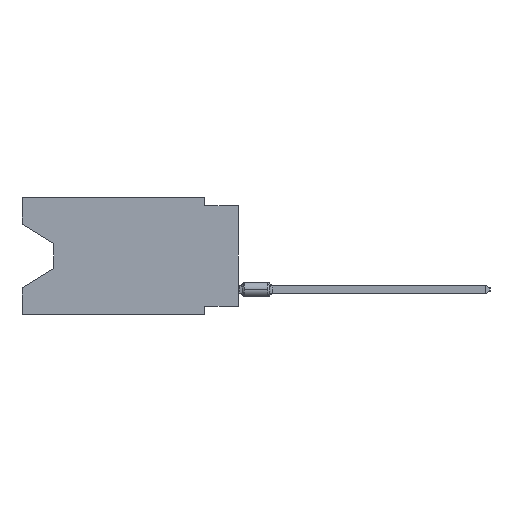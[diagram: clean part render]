
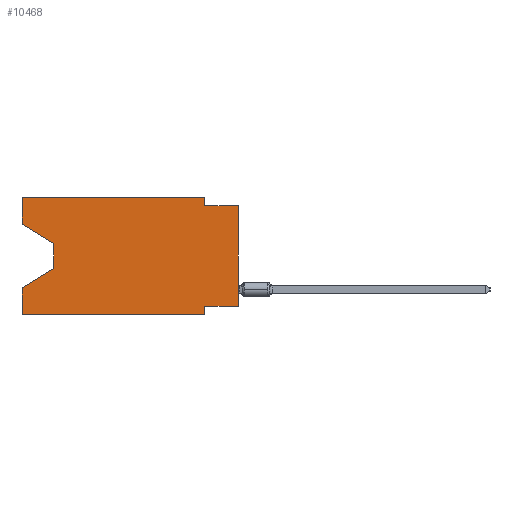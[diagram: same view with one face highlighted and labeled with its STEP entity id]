
A CAD part, left-side view. The second image highlights one B-rep face of the part: STEP entity #10468.
In plain terms, the highlighted planar face has unit normal (-1, 0, 0).
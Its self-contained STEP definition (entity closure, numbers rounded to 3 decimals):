
#1306 = EDGE_CURVE ( 'NONE', #19999, #4878, #35675, .T. ) ;
#1362 = DIRECTION ( 'NONE',  ( 0., 0., -1. ) ) ;
#1795 = VERTEX_POINT ( 'NONE', #6990 ) ;
#1924 = LINE ( 'NONE', #17501, #7468 ) ;
#2121 = DIRECTION ( 'NONE',  ( 0., 0., -1. ) ) ;
#3189 = CARTESIAN_POINT ( 'NONE',  ( 0., 0., 0. ) ) ;
#3445 = VERTEX_POINT ( 'NONE', #20941 ) ;
#3462 = LINE ( 'NONE', #12535, #15370 ) ;
#3590 = EDGE_CURVE ( 'NONE', #22829, #10053, #12602, .T. ) ;
#3717 = CARTESIAN_POINT ( 'NONE',  ( 0., 16.383, -8.89 ) ) ;
#4455 = LINE ( 'NONE', #10248, #30236 ) ;
#4628 = ORIENTED_EDGE ( 'NONE', *, *, #26332, .F. ) ;
#4878 = VERTEX_POINT ( 'NONE', #6322 ) ;
#4964 = EDGE_CURVE ( 'NONE', #11980, #38123, #12509, .T. ) ;
#5259 = CARTESIAN_POINT ( 'NONE',  ( 0., 2.54, -8.89 ) ) ;
#6066 = DIRECTION ( 'NONE',  ( 0., 0., 1. ) ) ;
#6203 = CARTESIAN_POINT ( 'NONE',  ( 0., 16.383, 0. ) ) ;
#6322 = CARTESIAN_POINT ( 'NONE',  ( 0., 0., -0.635 ) ) ;
#6726 = ORIENTED_EDGE ( 'NONE', *, *, #31662, .T. ) ;
#6990 = CARTESIAN_POINT ( 'NONE',  ( 0., 13.97, -5.385 ) ) ;
#6999 = DIRECTION ( 'NONE',  ( 0., -0.855, -0.519 ) ) ;
#7286 = CARTESIAN_POINT ( 'NONE',  ( 0., 16.383, -8.89 ) ) ;
#7453 = EDGE_CURVE ( 'NONE', #12518, #3445, #3462, .T. ) ;
#7468 = VECTOR ( 'NONE', #13704, 1000. ) ;
#7563 = CARTESIAN_POINT ( 'NONE',  ( 0., 16.383, 0. ) ) ;
#7879 = EDGE_CURVE ( 'NONE', #3445, #4878, #4455, .T. ) ;
#8936 = DIRECTION ( 'NONE',  ( 0., -1., 0. ) ) ;
#9057 = DIRECTION ( 'NONE',  ( 0., 0., -1. ) ) ;
#9687 = ORIENTED_EDGE ( 'NONE', *, *, #22630, .T. ) ;
#10053 = VERTEX_POINT ( 'NONE', #10497 ) ;
#10248 = CARTESIAN_POINT ( 'NONE',  ( 0., 0., -0.635 ) ) ;
#10468 = ADVANCED_FACE ( 'NONE', ( #37156 ), #30986, .F. ) ;
#10497 = CARTESIAN_POINT ( 'NONE',  ( 0., 13.97, -3.505 ) ) ;
#10500 = CARTESIAN_POINT ( 'NONE',  ( 0., 16.383, 0. ) ) ;
#10633 = DIRECTION ( 'NONE',  ( 1., 0., 0. ) ) ;
#11980 = VERTEX_POINT ( 'NONE', #3717 ) ;
#12202 = EDGE_LOOP ( 'NONE', ( #35691, #9687, #6726, #4628, #15227, #14943, #29211, #17017, #16393, #34634, #17916, #19439 ) ) ;
#12509 = LINE ( 'NONE', #7286, #16531 ) ;
#12518 = VERTEX_POINT ( 'NONE', #31122 ) ;
#12535 = CARTESIAN_POINT ( 'NONE',  ( 0., 2.54, 0. ) ) ;
#12602 = LINE ( 'NONE', #27507, #20723 ) ;
#13704 = DIRECTION ( 'NONE',  ( 0., 1., 0. ) ) ;
#14046 = VERTEX_POINT ( 'NONE', #27068 ) ;
#14943 = ORIENTED_EDGE ( 'NONE', *, *, #32409, .F. ) ;
#15227 = ORIENTED_EDGE ( 'NONE', *, *, #4964, .T. ) ;
#15370 = VECTOR ( 'NONE', #9057, 1000. ) ;
#15767 = VERTEX_POINT ( 'NONE', #17776 ) ;
#16393 = ORIENTED_EDGE ( 'NONE', *, *, #7879, .F. ) ;
#16439 = CARTESIAN_POINT ( 'NONE',  ( 0., 2.54, -8.89 ) ) ;
#16447 = DIRECTION ( 'NONE',  ( 0., -1., 0. ) ) ;
#16531 = VECTOR ( 'NONE', #36876, 1000. ) ;
#17017 = ORIENTED_EDGE ( 'NONE', *, *, #1306, .T. ) ;
#17078 = DIRECTION ( 'NONE',  ( 0., 0.855, -0.519 ) ) ;
#17501 = CARTESIAN_POINT ( 'NONE',  ( 0., 0., -8.255 ) ) ;
#17776 = CARTESIAN_POINT ( 'NONE',  ( 0., 16.383, -6.852 ) ) ;
#17916 = ORIENTED_EDGE ( 'NONE', *, *, #34792, .F. ) ;
#19439 = ORIENTED_EDGE ( 'NONE', *, *, #38060, .F. ) ;
#19814 = VECTOR ( 'NONE', #17078, 1000. ) ;
#19999 = VERTEX_POINT ( 'NONE', #29539 ) ;
#20723 = VECTOR ( 'NONE', #6999, 1000. ) ;
#20869 = CARTESIAN_POINT ( 'NONE',  ( 0., 16.383, -2.038 ) ) ;
#20917 = LINE ( 'NONE', #6203, #35139 ) ;
#20941 = CARTESIAN_POINT ( 'NONE',  ( 0., 2.54, -0.635 ) ) ;
#21034 = VECTOR ( 'NONE', #37204, 1000. ) ;
#22629 = CARTESIAN_POINT ( 'NONE',  ( 0., 13.97, -3.505 ) ) ;
#22630 = EDGE_CURVE ( 'NONE', #10053, #1795, #36245, .T. ) ;
#22829 = VERTEX_POINT ( 'NONE', #20869 ) ;
#25506 = VECTOR ( 'NONE', #6066, 1000. ) ;
#26324 = DIRECTION ( 'NONE',  ( 0., 0., 1. ) ) ;
#26332 = EDGE_CURVE ( 'NONE', #11980, #15767, #20917, .T. ) ;
#26561 = CARTESIAN_POINT ( 'NONE',  ( 0., 16.383, 0. ) ) ;
#27068 = CARTESIAN_POINT ( 'NONE',  ( 0., 16.383, 0. ) ) ;
#27507 = CARTESIAN_POINT ( 'NONE',  ( 0., 16.383, -2.038 ) ) ;
#28712 = LINE ( 'NONE', #38152, #19814 ) ;
#29211 = ORIENTED_EDGE ( 'NONE', *, *, #31299, .F. ) ;
#29539 = CARTESIAN_POINT ( 'NONE',  ( 0., 0., -8.255 ) ) ;
#30236 = VECTOR ( 'NONE', #16447, 1000. ) ;
#30766 = VECTOR ( 'NONE', #8936, 1000. ) ;
#30955 = LINE ( 'NONE', #16439, #32209 ) ;
#30986 = PLANE ( 'NONE',  #36577 ) ;
#31122 = CARTESIAN_POINT ( 'NONE',  ( 0., 2.54, 0. ) ) ;
#31299 = EDGE_CURVE ( 'NONE', #19999, #34408, #1924, .T. ) ;
#31662 = EDGE_CURVE ( 'NONE', #1795, #15767, #28712, .T. ) ;
#32209 = VECTOR ( 'NONE', #1362, 1000. ) ;
#32409 = EDGE_CURVE ( 'NONE', #34408, #38123, #30955, .T. ) ;
#34408 = VERTEX_POINT ( 'NONE', #35692 ) ;
#34435 = DIRECTION ( 'NONE',  ( 0., 0., -1. ) ) ;
#34634 = ORIENTED_EDGE ( 'NONE', *, *, #7453, .F. ) ;
#34792 = EDGE_CURVE ( 'NONE', #14046, #12518, #35443, .T. ) ;
#34943 = VECTOR ( 'NONE', #2121, 1000. ) ;
#35139 = VECTOR ( 'NONE', #26324, 1000. ) ;
#35443 = LINE ( 'NONE', #26561, #30766 ) ;
#35675 = LINE ( 'NONE', #3189, #25506 ) ;
#35691 = ORIENTED_EDGE ( 'NONE', *, *, #3590, .T. ) ;
#35692 = CARTESIAN_POINT ( 'NONE',  ( 0., 2.54, -8.255 ) ) ;
#36245 = LINE ( 'NONE', #22629, #34943 ) ;
#36577 = AXIS2_PLACEMENT_3D ( 'NONE', #7563, #10633, #34435 ) ;
#36876 = DIRECTION ( 'NONE',  ( 0., -1., 0. ) ) ;
#37018 = LINE ( 'NONE', #10500, #21034 ) ;
#37156 = FACE_OUTER_BOUND ( 'NONE', #12202, .T. ) ;
#37204 = DIRECTION ( 'NONE',  ( 0., 0., 1. ) ) ;
#38060 = EDGE_CURVE ( 'NONE', #22829, #14046, #37018, .T. ) ;
#38123 = VERTEX_POINT ( 'NONE', #5259 ) ;
#38152 = CARTESIAN_POINT ( 'NONE',  ( 0., 13.97, -5.385 ) ) ;
